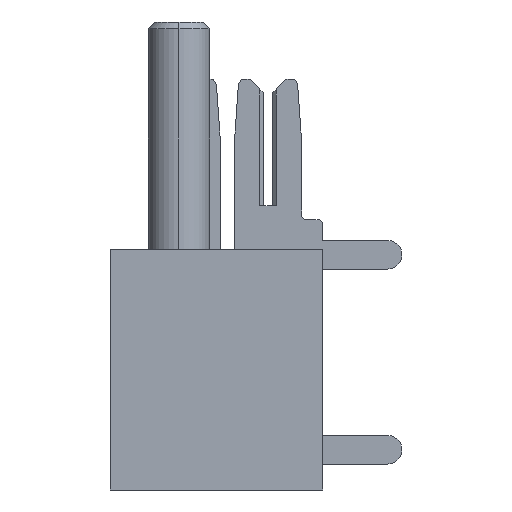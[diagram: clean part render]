
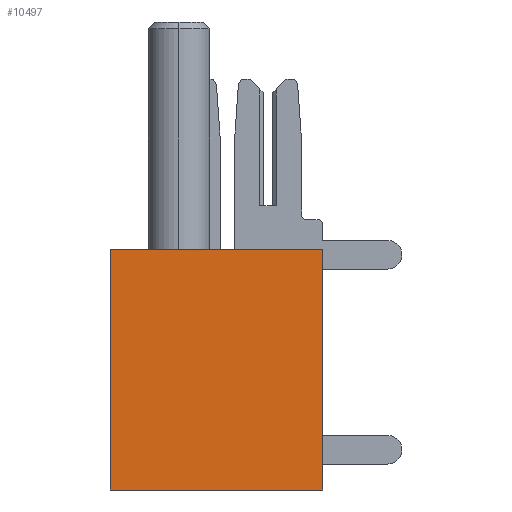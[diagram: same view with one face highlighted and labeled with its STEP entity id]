
A CAD part, left-side view. The second image highlights one B-rep face of the part: STEP entity #10497.
In plain terms, the highlighted planar face has unit normal (-1, 0, 0).
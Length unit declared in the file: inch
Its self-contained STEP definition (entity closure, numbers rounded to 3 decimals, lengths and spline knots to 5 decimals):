
#398 = VERTEX_POINT ( 'NONE', #11148 ) ;
#851 = CARTESIAN_POINT ( 'NONE',  ( 0., 0., -0.37 ) ) ;
#1235 = AXIS2_PLACEMENT_3D ( 'NONE', #2651, #6095, #6973 ) ;
#1439 = VERTEX_POINT ( 'NONE', #7071 ) ;
#2651 = CARTESIAN_POINT ( 'NONE',  ( 0., 0., -0.37 ) ) ;
#3486 = LINE ( 'NONE', #8501, #10250 ) ;
#3822 = VECTOR ( 'NONE', #7895, 39.37008 ) ;
#4168 = EDGE_CURVE ( 'NONE', #1439, #9541, #5065, .T. ) ;
#4210 = EDGE_LOOP ( 'NONE', ( #4945, #11269, #8841, #8606 ) ) ;
#4231 = PLANE ( 'NONE',  #1235 ) ;
#4429 = VERTEX_POINT ( 'NONE', #9082 ) ;
#4945 = ORIENTED_EDGE ( 'NONE', *, *, #10827, .F. ) ;
#5065 = LINE ( 'NONE', #851, #3822 ) ;
#5539 = DIRECTION ( 'NONE',  ( 0., -1., 0. ) ) ;
#5653 = CARTESIAN_POINT ( 'NONE',  ( 0., 0., 0. ) ) ;
#5956 = CARTESIAN_POINT ( 'NONE',  ( 0., 0., 0. ) ) ;
#6095 = DIRECTION ( 'NONE',  ( -1., 0., 0. ) ) ;
#6627 = VECTOR ( 'NONE', #5539, 39.37008 ) ;
#6916 = LINE ( 'NONE', #5653, #6627 ) ;
#6973 = DIRECTION ( 'NONE',  ( 0., 0., 1. ) ) ;
#7071 = CARTESIAN_POINT ( 'NONE',  ( 0., 0., -0.37 ) ) ;
#7884 = FACE_OUTER_BOUND ( 'NONE', #4210, .T. ) ;
#7895 = DIRECTION ( 'NONE',  ( 0., 0., 1. ) ) ;
#8005 = LINE ( 'NONE', #10485, #9398 ) ;
#8501 = CARTESIAN_POINT ( 'NONE',  ( 0., 0.327, -0.37 ) ) ;
#8606 = ORIENTED_EDGE ( 'NONE', *, *, #4168, .T. ) ;
#8746 = EDGE_CURVE ( 'NONE', #4429, #398, #3486, .T. ) ;
#8841 = ORIENTED_EDGE ( 'NONE', *, *, #9687, .T. ) ;
#9082 = CARTESIAN_POINT ( 'NONE',  ( 0., 0.327, -0.37 ) ) ;
#9398 = VECTOR ( 'NONE', #11374, 39.37008 ) ;
#9541 = VERTEX_POINT ( 'NONE', #5956 ) ;
#9687 = EDGE_CURVE ( 'NONE', #4429, #1439, #8005, .T. ) ;
#10250 = VECTOR ( 'NONE', #11122, 39.37008 ) ;
#10485 = CARTESIAN_POINT ( 'NONE',  ( 0., 0., -0.37 ) ) ;
#10497 = ADVANCED_FACE ( 'NONE', ( #7884 ), #4231, .T. ) ;
#10827 = EDGE_CURVE ( 'NONE', #398, #9541, #6916, .T. ) ;
#11122 = DIRECTION ( 'NONE',  ( 0., 0., 1. ) ) ;
#11148 = CARTESIAN_POINT ( 'NONE',  ( 0., 0.327, 0. ) ) ;
#11269 = ORIENTED_EDGE ( 'NONE', *, *, #8746, .F. ) ;
#11374 = DIRECTION ( 'NONE',  ( 0., -1., 0. ) ) ;
